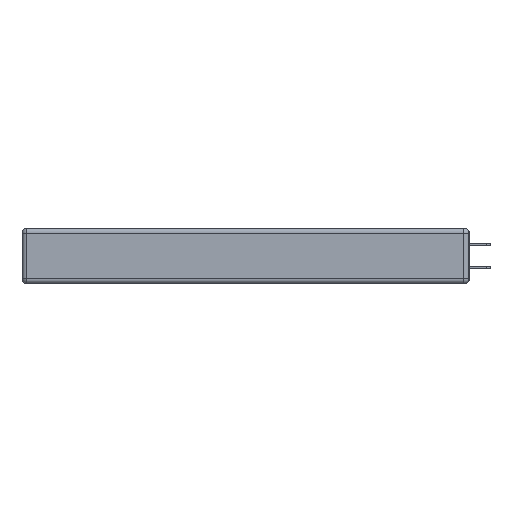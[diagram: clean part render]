
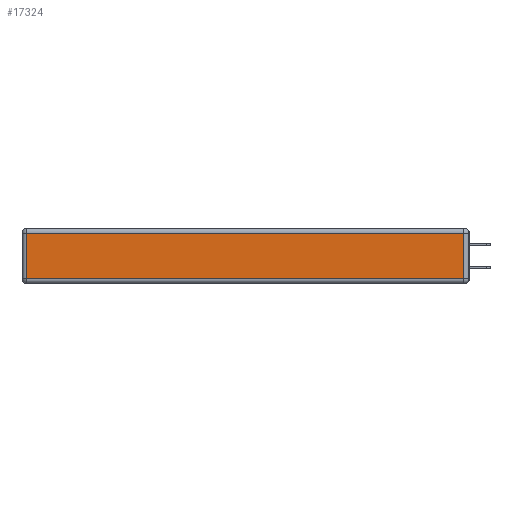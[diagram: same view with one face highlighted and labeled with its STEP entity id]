
A CAD part, left-side view. The second image highlights one B-rep face of the part: STEP entity #17324.
In plain terms, the highlighted planar face has unit normal (-1, 0, 0).
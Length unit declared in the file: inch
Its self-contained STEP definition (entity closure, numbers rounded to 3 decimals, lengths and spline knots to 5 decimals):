
#588 = DIRECTION ( 'NONE',  ( 0., 1., 0. ) ) ;
#926 = CARTESIAN_POINT ( 'NONE',  ( 0., 0., -0.343 ) ) ;
#1309 = VERTEX_POINT ( 'NONE', #5519 ) ;
#1338 = LINE ( 'NONE', #15185, #4227 ) ;
#1349 = ORIENTED_EDGE ( 'NONE', *, *, #21669, .T. ) ;
#1713 = VECTOR ( 'NONE', #13553, 39.37008 ) ;
#3677 = EDGE_LOOP ( 'NONE', ( #17838, #4328, #11628, #1349 ) ) ;
#4227 = VECTOR ( 'NONE', #588, 39.37008 ) ;
#4328 = ORIENTED_EDGE ( 'NONE', *, *, #10246, .T. ) ;
#5519 = CARTESIAN_POINT ( 'NONE',  ( 0., 0.03, -0.03 ) ) ;
#7210 = EDGE_CURVE ( 'NONE', #1309, #17006, #1338, .T. ) ;
#8330 = CARTESIAN_POINT ( 'NONE',  ( 0., 0., -0.313 ) ) ;
#9500 = VERTEX_POINT ( 'NONE', #16653 ) ;
#9964 = CARTESIAN_POINT ( 'NONE',  ( 0., 2.72, -0.343 ) ) ;
#10130 = DIRECTION ( 'NONE',  ( 0., 0., -1. ) ) ;
#10246 = EDGE_CURVE ( 'NONE', #9500, #1309, #20947, .T. ) ;
#10658 = CARTESIAN_POINT ( 'NONE',  ( 0., 0.03, -0.343 ) ) ;
#11391 = VERTEX_POINT ( 'NONE', #13350 ) ;
#11628 = ORIENTED_EDGE ( 'NONE', *, *, #7210, .T. ) ;
#12756 = LINE ( 'NONE', #8330, #20062 ) ;
#12787 = EDGE_CURVE ( 'NONE', #11391, #9500, #12756, .T. ) ;
#13350 = CARTESIAN_POINT ( 'NONE',  ( 0., 2.72, -0.313 ) ) ;
#13553 = DIRECTION ( 'NONE',  ( 0., 0., 1. ) ) ;
#13635 = DIRECTION ( 'NONE',  ( 0., -1., 0. ) ) ;
#15185 = CARTESIAN_POINT ( 'NONE',  ( 0., 2.75, -0.03 ) ) ;
#16424 = FACE_OUTER_BOUND ( 'NONE', #3677, .T. ) ;
#16653 = CARTESIAN_POINT ( 'NONE',  ( 0., 0.03, -0.313 ) ) ;
#16818 = VECTOR ( 'NONE', #10130, 39.37008 ) ;
#16830 = CARTESIAN_POINT ( 'NONE',  ( 0., 2.72, -0.03 ) ) ;
#17006 = VERTEX_POINT ( 'NONE', #16830 ) ;
#17324 = ADVANCED_FACE ( 'NONE', ( #16424 ), #21248, .T. ) ;
#17838 = ORIENTED_EDGE ( 'NONE', *, *, #12787, .T. ) ;
#20062 = VECTOR ( 'NONE', #13635, 39.37008 ) ;
#20947 = LINE ( 'NONE', #10658, #1713 ) ;
#21173 = DIRECTION ( 'NONE',  ( -1., 0., 0. ) ) ;
#21248 = PLANE ( 'NONE',  #21280 ) ;
#21280 = AXIS2_PLACEMENT_3D ( 'NONE', #926, #21173, #22973 ) ;
#21669 = EDGE_CURVE ( 'NONE', #17006, #11391, #22926, .T. ) ;
#22926 = LINE ( 'NONE', #9964, #16818 ) ;
#22973 = DIRECTION ( 'NONE',  ( 0., 0., 1. ) ) ;
